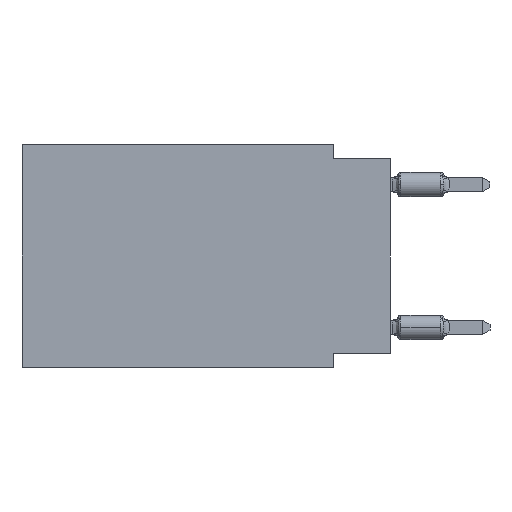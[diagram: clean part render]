
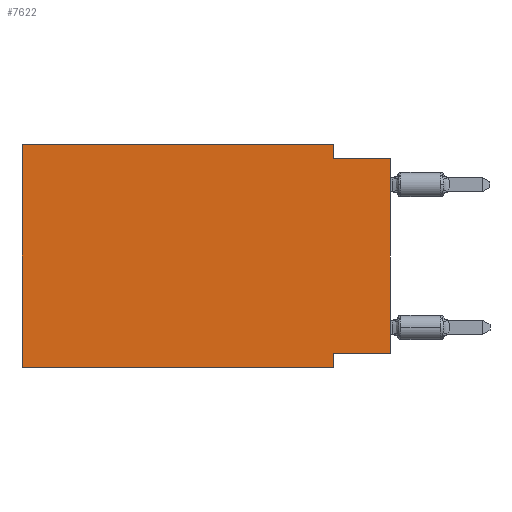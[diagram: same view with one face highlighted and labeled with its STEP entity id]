
A CAD part, left-side view. The second image highlights one B-rep face of the part: STEP entity #7622.
In plain terms, the highlighted planar face has unit normal (-1, 0, 0).
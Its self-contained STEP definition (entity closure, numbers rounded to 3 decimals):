
#59 = EDGE_CURVE ( 'NONE', #11188, #3638, #2030, .T. ) ;
#521 = VERTEX_POINT ( 'NONE', #9881 ) ;
#1060 = EDGE_CURVE ( 'NONE', #5951, #17255, #2860, .T. ) ;
#1280 = EDGE_CURVE ( 'NONE', #3638, #17255, #19012, .T. ) ;
#2030 = LINE ( 'NONE', #4957, #13622 ) ;
#2173 = CARTESIAN_POINT ( 'NONE',  ( 0., 2.54, -9.271 ) ) ;
#2860 = LINE ( 'NONE', #15484, #4311 ) ;
#3512 = LINE ( 'NONE', #10999, #12408 ) ;
#3638 = VERTEX_POINT ( 'NONE', #14302 ) ;
#4311 = VECTOR ( 'NONE', #5990, 1000. ) ;
#4805 = LINE ( 'NONE', #6424, #14963 ) ;
#4957 = CARTESIAN_POINT ( 'NONE',  ( 0., 2.54, 0. ) ) ;
#5016 = DIRECTION ( 'NONE',  ( 0., 1., 0. ) ) ;
#5671 = ORIENTED_EDGE ( 'NONE', *, *, #7695, .F. ) ;
#5951 = VERTEX_POINT ( 'NONE', #18035 ) ;
#5990 = DIRECTION ( 'NONE',  ( 0., 0., 1. ) ) ;
#6424 = CARTESIAN_POINT ( 'NONE',  ( 0., 16.383, 0. ) ) ;
#6494 = LINE ( 'NONE', #11134, #10459 ) ;
#6578 = DIRECTION ( 'NONE',  ( 0., 0., -1. ) ) ;
#7410 = EDGE_LOOP ( 'NONE', ( #16606, #18993, #17381, #5671, #15754, #15935, #11554, #19458 ) ) ;
#7622 = ADVANCED_FACE ( 'NONE', ( #12083 ), #13696, .F. ) ;
#7657 = LINE ( 'NONE', #9268, #8966 ) ;
#7695 = EDGE_CURVE ( 'NONE', #8335, #11188, #6494, .T. ) ;
#7749 = DIRECTION ( 'NONE',  ( 0., 0., 1. ) ) ;
#7875 = DIRECTION ( 'NONE',  ( 0., -1., 0. ) ) ;
#8196 = AXIS2_PLACEMENT_3D ( 'NONE', #16723, #17391, #16827 ) ;
#8335 = VERTEX_POINT ( 'NONE', #8667 ) ;
#8667 = CARTESIAN_POINT ( 'NONE',  ( 0., 16.383, 0. ) ) ;
#8966 = VECTOR ( 'NONE', #5016, 1000. ) ;
#9020 = VERTEX_POINT ( 'NONE', #2173 ) ;
#9268 = CARTESIAN_POINT ( 'NONE',  ( 0., 0., -9.271 ) ) ;
#9878 = CARTESIAN_POINT ( 'NONE',  ( 0., 2.54, -9.906 ) ) ;
#9881 = CARTESIAN_POINT ( 'NONE',  ( 0., 2.54, -9.906 ) ) ;
#10166 = LINE ( 'NONE', #9878, #15980 ) ;
#10175 = EDGE_CURVE ( 'NONE', #14900, #521, #3512, .T. ) ;
#10459 = VECTOR ( 'NONE', #17296, 1000. ) ;
#10999 = CARTESIAN_POINT ( 'NONE',  ( 0., 16.383, -9.906 ) ) ;
#11134 = CARTESIAN_POINT ( 'NONE',  ( 0., 16.383, 0. ) ) ;
#11188 = VERTEX_POINT ( 'NONE', #17974 ) ;
#11322 = CARTESIAN_POINT ( 'NONE',  ( 0., 0., -0.635 ) ) ;
#11554 = ORIENTED_EDGE ( 'NONE', *, *, #11624, .F. ) ;
#11624 = EDGE_CURVE ( 'NONE', #9020, #521, #10166, .T. ) ;
#12083 = FACE_OUTER_BOUND ( 'NONE', #7410, .T. ) ;
#12408 = VECTOR ( 'NONE', #7875, 1000. ) ;
#13622 = VECTOR ( 'NONE', #6578, 1000. ) ;
#13696 = PLANE ( 'NONE',  #8196 ) ;
#14302 = CARTESIAN_POINT ( 'NONE',  ( 0., 2.54, -0.635 ) ) ;
#14900 = VERTEX_POINT ( 'NONE', #18163 ) ;
#14963 = VECTOR ( 'NONE', #7749, 1000. ) ;
#15047 = EDGE_CURVE ( 'NONE', #5951, #9020, #7657, .T. ) ;
#15484 = CARTESIAN_POINT ( 'NONE',  ( 0., 0., 0. ) ) ;
#15688 = DIRECTION ( 'NONE',  ( 0., -1., 0. ) ) ;
#15754 = ORIENTED_EDGE ( 'NONE', *, *, #17543, .F. ) ;
#15935 = ORIENTED_EDGE ( 'NONE', *, *, #10175, .T. ) ;
#15980 = VECTOR ( 'NONE', #16341, 1000. ) ;
#15982 = CARTESIAN_POINT ( 'NONE',  ( 0., 0., -0.635 ) ) ;
#16341 = DIRECTION ( 'NONE',  ( 0., 0., -1. ) ) ;
#16606 = ORIENTED_EDGE ( 'NONE', *, *, #1060, .T. ) ;
#16723 = CARTESIAN_POINT ( 'NONE',  ( 0., 16.383, 0. ) ) ;
#16827 = DIRECTION ( 'NONE',  ( 0., 0., -1. ) ) ;
#17255 = VERTEX_POINT ( 'NONE', #11322 ) ;
#17296 = DIRECTION ( 'NONE',  ( 0., -1., 0. ) ) ;
#17381 = ORIENTED_EDGE ( 'NONE', *, *, #59, .F. ) ;
#17391 = DIRECTION ( 'NONE',  ( 1., 0., 0. ) ) ;
#17540 = VECTOR ( 'NONE', #15688, 1000. ) ;
#17543 = EDGE_CURVE ( 'NONE', #14900, #8335, #4805, .T. ) ;
#17974 = CARTESIAN_POINT ( 'NONE',  ( 0., 2.54, 0. ) ) ;
#18035 = CARTESIAN_POINT ( 'NONE',  ( 0., 0., -9.271 ) ) ;
#18163 = CARTESIAN_POINT ( 'NONE',  ( 0., 16.383, -9.906 ) ) ;
#18993 = ORIENTED_EDGE ( 'NONE', *, *, #1280, .F. ) ;
#19012 = LINE ( 'NONE', #15982, #17540 ) ;
#19458 = ORIENTED_EDGE ( 'NONE', *, *, #15047, .F. ) ;
